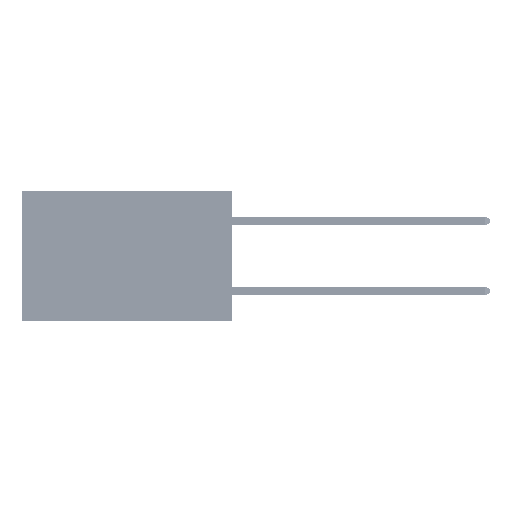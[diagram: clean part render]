
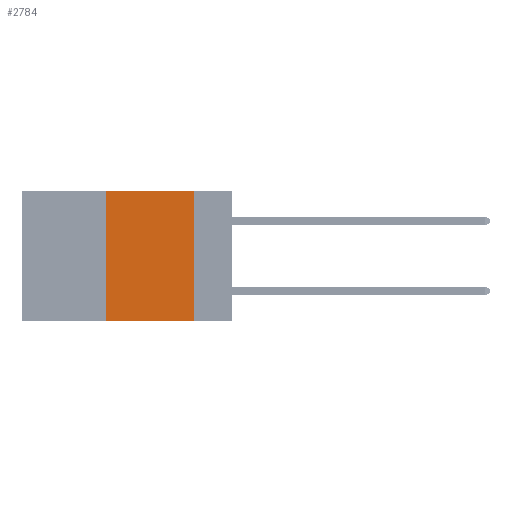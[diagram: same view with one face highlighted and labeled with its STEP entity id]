
A CAD part, left-side view. The second image highlights one B-rep face of the part: STEP entity #2784.
In plain terms, the highlighted planar face has unit normal (-1, 0, 0).
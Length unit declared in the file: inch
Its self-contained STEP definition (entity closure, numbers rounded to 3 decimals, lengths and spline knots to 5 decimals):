
#1404 = DIRECTION ( 'NONE',  ( 1., 0., 0. ) ) ;
#1864 = VERTEX_POINT ( 'NONE', #11100 ) ;
#1989 = CARTESIAN_POINT ( 'NONE',  ( 0., 0.36, -0.37 ) ) ;
#2784 = ADVANCED_FACE ( 'NONE', ( #41314 ), #17730, .F. ) ;
#3390 = VECTOR ( 'NONE', #22070, 39.37008 ) ;
#4141 = VERTEX_POINT ( 'NONE', #28381 ) ;
#5500 = CARTESIAN_POINT ( 'NONE',  ( 0., 0.11, 0. ) ) ;
#6318 = DIRECTION ( 'NONE',  ( 0., 0., 1. ) ) ;
#8015 = ORIENTED_EDGE ( 'NONE', *, *, #16993, .F. ) ;
#9420 = VECTOR ( 'NONE', #17831, 39.37008 ) ;
#11100 = CARTESIAN_POINT ( 'NONE',  ( 0., 0.11, -0.37 ) ) ;
#16376 = DIRECTION ( 'NONE',  ( 0., -1., 0. ) ) ;
#16993 = EDGE_CURVE ( 'NONE', #29625, #1864, #20454, .T. ) ;
#17326 = LINE ( 'NONE', #36274, #25119 ) ;
#17730 = PLANE ( 'NONE',  #22235 ) ;
#17831 = DIRECTION ( 'NONE',  ( 0., 0., -1. ) ) ;
#20454 = LINE ( 'NONE', #5500, #9420 ) ;
#22070 = DIRECTION ( 'NONE',  ( 0., -1., 0. ) ) ;
#22235 = AXIS2_PLACEMENT_3D ( 'NONE', #23162, #1404, #26064 ) ;
#22655 = CARTESIAN_POINT ( 'NONE',  ( 0., 0.36, 0. ) ) ;
#23162 = CARTESIAN_POINT ( 'NONE',  ( 0., 0.6, 0. ) ) ;
#23501 = EDGE_CURVE ( 'NONE', #29538, #1864, #17326, .T. ) ;
#25119 = VECTOR ( 'NONE', #16376, 39.37008 ) ;
#25454 = LINE ( 'NONE', #38126, #3390 ) ;
#26064 = DIRECTION ( 'NONE',  ( 0., 0., -1. ) ) ;
#28381 = CARTESIAN_POINT ( 'NONE',  ( 0., 0.36, 0. ) ) ;
#29538 = VERTEX_POINT ( 'NONE', #1989 ) ;
#29625 = VERTEX_POINT ( 'NONE', #52292 ) ;
#33349 = VECTOR ( 'NONE', #6318, 39.37008 ) ;
#34635 = LINE ( 'NONE', #22655, #33349 ) ;
#36274 = CARTESIAN_POINT ( 'NONE',  ( 0., 0.6, -0.37 ) ) ;
#37525 = ORIENTED_EDGE ( 'NONE', *, *, #50667, .F. ) ;
#38126 = CARTESIAN_POINT ( 'NONE',  ( 0., 0.6, 0. ) ) ;
#39191 = EDGE_CURVE ( 'NONE', #4141, #29625, #25454, .T. ) ;
#41314 = FACE_OUTER_BOUND ( 'NONE', #51170, .T. ) ;
#50667 = EDGE_CURVE ( 'NONE', #29538, #4141, #34635, .T. ) ;
#51050 = ORIENTED_EDGE ( 'NONE', *, *, #39191, .F. ) ;
#51170 = EDGE_LOOP ( 'NONE', ( #8015, #51050, #37525, #52469 ) ) ;
#52292 = CARTESIAN_POINT ( 'NONE',  ( 0., 0.11, 0. ) ) ;
#52469 = ORIENTED_EDGE ( 'NONE', *, *, #23501, .T. ) ;
